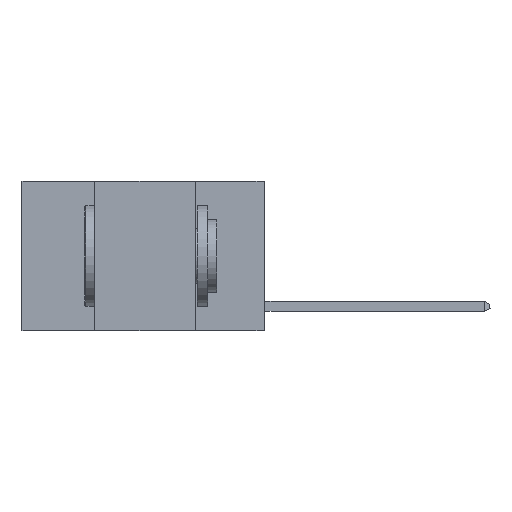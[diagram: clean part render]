
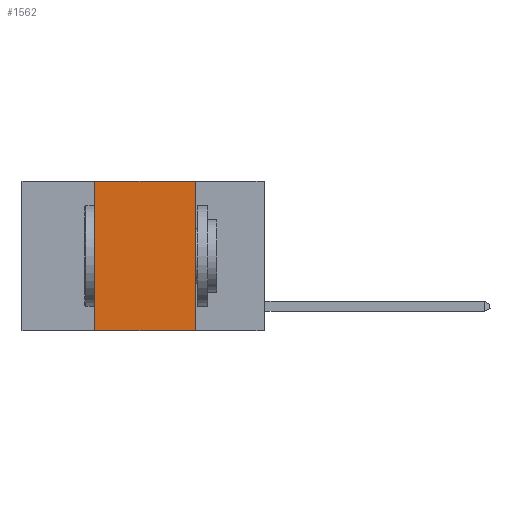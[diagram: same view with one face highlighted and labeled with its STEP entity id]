
A CAD part, left-side view. The second image highlights one B-rep face of the part: STEP entity #1562.
In plain terms, the highlighted planar face has unit normal (-1, 0, 0).
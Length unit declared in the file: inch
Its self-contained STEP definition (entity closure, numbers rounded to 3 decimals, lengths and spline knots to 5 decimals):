
#229 = LINE ( 'NONE', #6107, #12419 ) ;
#379 = DIRECTION ( 'NONE',  ( 1., 0., 0. ) ) ;
#1065 = DIRECTION ( 'NONE',  ( 0., 0., 1. ) ) ;
#1264 = VERTEX_POINT ( 'NONE', #13670 ) ;
#1401 = CARTESIAN_POINT ( 'NONE',  ( 0., 0.17, 0. ) ) ;
#1562 = ADVANCED_FACE ( 'NONE', ( #7479 ), #9786, .F. ) ;
#1687 = ORIENTED_EDGE ( 'NONE', *, *, #4817, .T. ) ;
#1811 = EDGE_CURVE ( 'NONE', #11402, #1264, #8233, .T. ) ;
#2292 = CARTESIAN_POINT ( 'NONE',  ( 0., 0.42, 0. ) ) ;
#2909 = LINE ( 'NONE', #14624, #12204 ) ;
#3872 = CARTESIAN_POINT ( 'NONE',  ( 0., 0.6, 0. ) ) ;
#4817 = EDGE_CURVE ( 'NONE', #11183, #1264, #2909, .T. ) ;
#5707 = DIRECTION ( 'NONE',  ( 0., 0., -1. ) ) ;
#5718 = ORIENTED_EDGE ( 'NONE', *, *, #5788, .F. ) ;
#5788 = EDGE_CURVE ( 'NONE', #11183, #9564, #229, .T. ) ;
#6107 = CARTESIAN_POINT ( 'NONE',  ( 0., 0.42, 0. ) ) ;
#6111 = DIRECTION ( 'NONE',  ( 0., 0., -1. ) ) ;
#7032 = VECTOR ( 'NONE', #10244, 39.37008 ) ;
#7479 = FACE_OUTER_BOUND ( 'NONE', #9009, .T. ) ;
#8018 = CARTESIAN_POINT ( 'NONE',  ( 0., 0.6, 0. ) ) ;
#8087 = CARTESIAN_POINT ( 'NONE',  ( 0., 0.17, 0. ) ) ;
#8233 = LINE ( 'NONE', #8087, #15116 ) ;
#8656 = ORIENTED_EDGE ( 'NONE', *, *, #8725, .F. ) ;
#8725 = EDGE_CURVE ( 'NONE', #9564, #11402, #9254, .T. ) ;
#9009 = EDGE_LOOP ( 'NONE', ( #12715, #8656, #5718, #1687 ) ) ;
#9254 = LINE ( 'NONE', #8018, #7032 ) ;
#9564 = VERTEX_POINT ( 'NONE', #2292 ) ;
#9786 = PLANE ( 'NONE',  #14129 ) ;
#10244 = DIRECTION ( 'NONE',  ( 0., -1., 0. ) ) ;
#11183 = VERTEX_POINT ( 'NONE', #11189 ) ;
#11189 = CARTESIAN_POINT ( 'NONE',  ( 0., 0.42, -0.37 ) ) ;
#11402 = VERTEX_POINT ( 'NONE', #1401 ) ;
#12193 = DIRECTION ( 'NONE',  ( 0., -1., 0. ) ) ;
#12204 = VECTOR ( 'NONE', #12193, 39.37008 ) ;
#12419 = VECTOR ( 'NONE', #1065, 39.37008 ) ;
#12715 = ORIENTED_EDGE ( 'NONE', *, *, #1811, .F. ) ;
#13670 = CARTESIAN_POINT ( 'NONE',  ( 0., 0.17, -0.37 ) ) ;
#14129 = AXIS2_PLACEMENT_3D ( 'NONE', #3872, #379, #6111 ) ;
#14624 = CARTESIAN_POINT ( 'NONE',  ( 0., 0.6, -0.37 ) ) ;
#15116 = VECTOR ( 'NONE', #5707, 39.37008 ) ;
